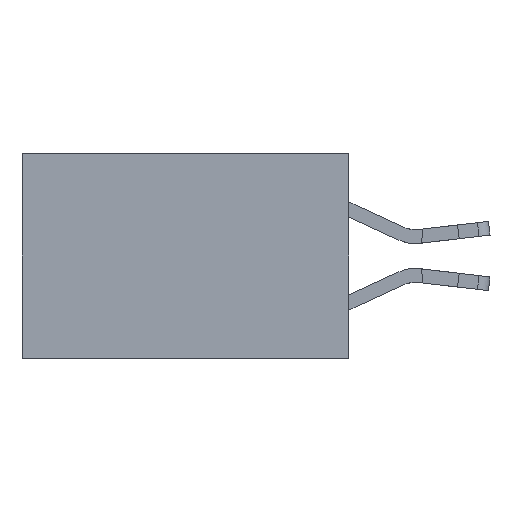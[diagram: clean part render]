
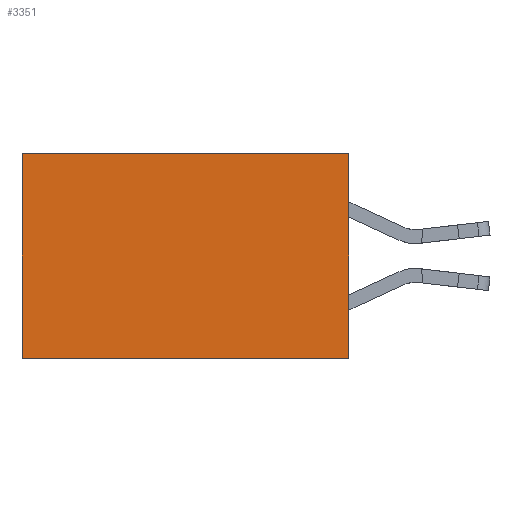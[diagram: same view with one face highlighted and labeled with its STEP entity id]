
A CAD part, left-side view. The second image highlights one B-rep face of the part: STEP entity #3351.
In plain terms, the highlighted planar face has unit normal (-1, 0, 0).
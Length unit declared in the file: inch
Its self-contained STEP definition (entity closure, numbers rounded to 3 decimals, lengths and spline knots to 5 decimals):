
#336 = VECTOR ( 'NONE', #2926, 39.37008 ) ;
#842 = LINE ( 'NONE', #3000, #336 ) ;
#852 = EDGE_CURVE ( 'NONE', #13917, #11780, #1167, .T. ) ;
#1154 = CARTESIAN_POINT ( 'NONE',  ( 0.277, 0.59, 0. ) ) ;
#1167 = LINE ( 'NONE', #15656, #4402 ) ;
#2926 = DIRECTION ( 'NONE',  ( 0., 1., 0. ) ) ;
#3000 = CARTESIAN_POINT ( 'NONE',  ( 0.277, 0., -0.37 ) ) ;
#3351 = ADVANCED_FACE ( 'NONE', ( #4747 ), #17289, .F. ) ;
#4402 = VECTOR ( 'NONE', #10027, 39.37008 ) ;
#4747 = FACE_OUTER_BOUND ( 'NONE', #10310, .T. ) ;
#5096 = DIRECTION ( 'NONE',  ( 0., 0., -1. ) ) ;
#5107 = VECTOR ( 'NONE', #5096, 39.37008 ) ;
#6287 = EDGE_CURVE ( 'NONE', #13917, #10445, #14838, .T. ) ;
#7443 = ORIENTED_EDGE ( 'NONE', *, *, #16181, .T. ) ;
#7554 = VECTOR ( 'NONE', #12011, 39.37008 ) ;
#7643 = CARTESIAN_POINT ( 'NONE',  ( 0.277, 0., -0.37 ) ) ;
#7763 = ORIENTED_EDGE ( 'NONE', *, *, #8858, .F. ) ;
#7778 = AXIS2_PLACEMENT_3D ( 'NONE', #15189, #15172, #17165 ) ;
#7834 = LINE ( 'NONE', #14616, #5107 ) ;
#8090 = ORIENTED_EDGE ( 'NONE', *, *, #852, .F. ) ;
#8858 = EDGE_CURVE ( 'NONE', #11780, #11484, #842, .T. ) ;
#9880 = CARTESIAN_POINT ( 'NONE',  ( 0.277, 0.59, -0.37 ) ) ;
#10027 = DIRECTION ( 'NONE',  ( 0., 0., -1. ) ) ;
#10310 = EDGE_LOOP ( 'NONE', ( #7443, #7763, #8090, #16432 ) ) ;
#10445 = VERTEX_POINT ( 'NONE', #1154 ) ;
#11484 = VERTEX_POINT ( 'NONE', #9880 ) ;
#11780 = VERTEX_POINT ( 'NONE', #7643 ) ;
#12011 = DIRECTION ( 'NONE',  ( 0., 1., 0. ) ) ;
#13917 = VERTEX_POINT ( 'NONE', #16224 ) ;
#14616 = CARTESIAN_POINT ( 'NONE',  ( 0.277, 0.59, -0.37 ) ) ;
#14838 = LINE ( 'NONE', #17182, #7554 ) ;
#15172 = DIRECTION ( 'NONE',  ( 1., 0., 0. ) ) ;
#15189 = CARTESIAN_POINT ( 'NONE',  ( 0.277, 0., -0.37 ) ) ;
#15656 = CARTESIAN_POINT ( 'NONE',  ( 0.277, 0., -0.37 ) ) ;
#16181 = EDGE_CURVE ( 'NONE', #10445, #11484, #7834, .T. ) ;
#16224 = CARTESIAN_POINT ( 'NONE',  ( 0.277, 0., 0. ) ) ;
#16432 = ORIENTED_EDGE ( 'NONE', *, *, #6287, .T. ) ;
#17165 = DIRECTION ( 'NONE',  ( 0., 0., -1. ) ) ;
#17182 = CARTESIAN_POINT ( 'NONE',  ( 0.277, 0., 0. ) ) ;
#17289 = PLANE ( 'NONE',  #7778 ) ;
